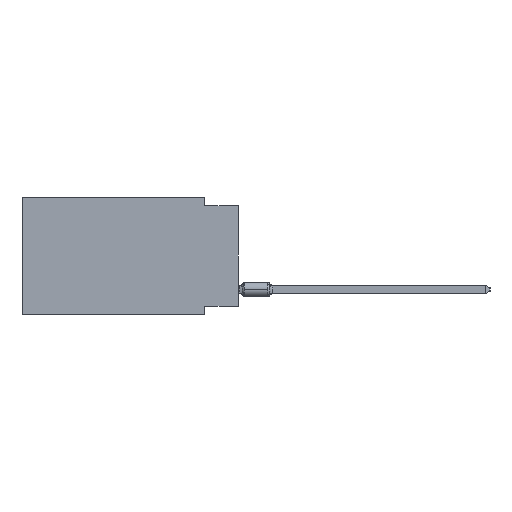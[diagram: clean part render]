
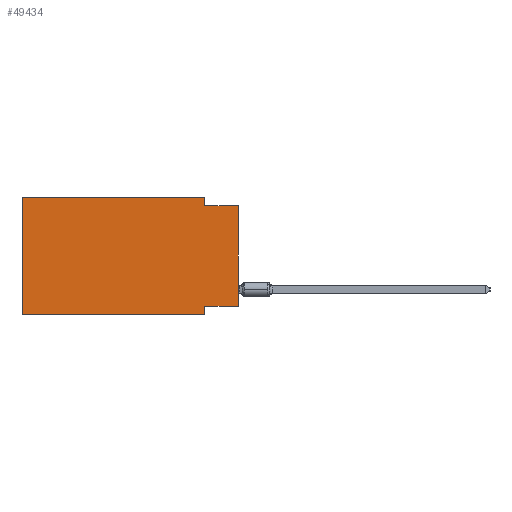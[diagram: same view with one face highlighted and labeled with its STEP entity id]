
A CAD part, left-side view. The second image highlights one B-rep face of the part: STEP entity #49434.
In plain terms, the highlighted planar face has unit normal (-1, 0, 0).
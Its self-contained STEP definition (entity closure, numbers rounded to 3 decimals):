
#2745 = DIRECTION ( 'NONE',  ( 0., -1., 0. ) ) ;
#3192 = ORIENTED_EDGE ( 'NONE', *, *, #61777, .T. ) ;
#5696 = ORIENTED_EDGE ( 'NONE', *, *, #51660, .F. ) ;
#6144 = VERTEX_POINT ( 'NONE', #36738 ) ;
#7599 = DIRECTION ( 'NONE',  ( 1., 0., 0. ) ) ;
#7860 = CARTESIAN_POINT ( 'NONE',  ( 0., 2.54, 0. ) ) ;
#9140 = CARTESIAN_POINT ( 'NONE',  ( 0., 2.54, -8.89 ) ) ;
#10076 = EDGE_CURVE ( 'NONE', #32012, #53193, #49525, .T. ) ;
#12968 = VECTOR ( 'NONE', #25764, 1000. ) ;
#13190 = AXIS2_PLACEMENT_3D ( 'NONE', #27248, #7599, #41908 ) ;
#13434 = LINE ( 'NONE', #22494, #43256 ) ;
#13563 = CARTESIAN_POINT ( 'NONE',  ( 0., 16.383, -8.89 ) ) ;
#13908 = CARTESIAN_POINT ( 'NONE',  ( 0., 0., -8.255 ) ) ;
#14457 = VECTOR ( 'NONE', #58638, 1000. ) ;
#14818 = DIRECTION ( 'NONE',  ( 0., -1., 0. ) ) ;
#14846 = LINE ( 'NONE', #33579, #31772 ) ;
#15227 = VERTEX_POINT ( 'NONE', #36261 ) ;
#16390 = VERTEX_POINT ( 'NONE', #13908 ) ;
#16767 = ORIENTED_EDGE ( 'NONE', *, *, #41672, .F. ) ;
#16909 = EDGE_CURVE ( 'NONE', #6144, #32012, #20112, .T. ) ;
#20112 = LINE ( 'NONE', #53565, #37125 ) ;
#20499 = CARTESIAN_POINT ( 'NONE',  ( 0., 0., -8.255 ) ) ;
#20774 = EDGE_CURVE ( 'NONE', #15227, #38412, #13434, .T. ) ;
#21414 = EDGE_CURVE ( 'NONE', #16390, #15227, #24565, .T. ) ;
#21467 = VECTOR ( 'NONE', #34677, 1000. ) ;
#22494 = CARTESIAN_POINT ( 'NONE',  ( 0., 2.54, -8.89 ) ) ;
#22847 = FACE_OUTER_BOUND ( 'NONE', #27957, .T. ) ;
#24565 = LINE ( 'NONE', #20499, #14457 ) ;
#25764 = DIRECTION ( 'NONE',  ( 0., 0., -1. ) ) ;
#27248 = CARTESIAN_POINT ( 'NONE',  ( 0., 16.383, 0. ) ) ;
#27957 = EDGE_LOOP ( 'NONE', ( #3192, #5696, #31625, #56081, #16767, #61664, #41090, #37866 ) ) ;
#31313 = DIRECTION ( 'NONE',  ( 0., 0., 1. ) ) ;
#31377 = CARTESIAN_POINT ( 'NONE',  ( 0., 16.383, -8.89 ) ) ;
#31625 = ORIENTED_EDGE ( 'NONE', *, *, #10076, .F. ) ;
#31772 = VECTOR ( 'NONE', #42969, 1000. ) ;
#31917 = PLANE ( 'NONE',  #13190 ) ;
#32012 = VERTEX_POINT ( 'NONE', #7860 ) ;
#33579 = CARTESIAN_POINT ( 'NONE',  ( 0., 0., -0.635 ) ) ;
#33860 = VECTOR ( 'NONE', #2745, 1000. ) ;
#34677 = DIRECTION ( 'NONE',  ( 0., 0., 1. ) ) ;
#35745 = CARTESIAN_POINT ( 'NONE',  ( 0., 2.54, 0. ) ) ;
#36261 = CARTESIAN_POINT ( 'NONE',  ( 0., 2.54, -8.255 ) ) ;
#36738 = CARTESIAN_POINT ( 'NONE',  ( 0., 16.383, 0. ) ) ;
#37125 = VECTOR ( 'NONE', #14818, 1000. ) ;
#37866 = ORIENTED_EDGE ( 'NONE', *, *, #21414, .F. ) ;
#38412 = VERTEX_POINT ( 'NONE', #9140 ) ;
#40692 = CARTESIAN_POINT ( 'NONE',  ( 0., 0., 0. ) ) ;
#40910 = VECTOR ( 'NONE', #31313, 1000. ) ;
#41090 = ORIENTED_EDGE ( 'NONE', *, *, #20774, .F. ) ;
#41672 = EDGE_CURVE ( 'NONE', #49804, #6144, #48441, .T. ) ;
#41908 = DIRECTION ( 'NONE',  ( 0., 0., -1. ) ) ;
#42969 = DIRECTION ( 'NONE',  ( 0., -1., 0. ) ) ;
#43256 = VECTOR ( 'NONE', #55942, 1000. ) ;
#44353 = CARTESIAN_POINT ( 'NONE',  ( 0., 16.383, 0. ) ) ;
#45091 = EDGE_CURVE ( 'NONE', #49804, #38412, #47283, .T. ) ;
#47137 = VERTEX_POINT ( 'NONE', #61657 ) ;
#47283 = LINE ( 'NONE', #13563, #33860 ) ;
#47431 = CARTESIAN_POINT ( 'NONE',  ( 0., 2.54, -0.635 ) ) ;
#48441 = LINE ( 'NONE', #44353, #21467 ) ;
#49434 = ADVANCED_FACE ( 'NONE', ( #22847 ), #31917, .F. ) ;
#49525 = LINE ( 'NONE', #35745, #12968 ) ;
#49804 = VERTEX_POINT ( 'NONE', #31377 ) ;
#51660 = EDGE_CURVE ( 'NONE', #53193, #47137, #14846, .T. ) ;
#53193 = VERTEX_POINT ( 'NONE', #47431 ) ;
#53565 = CARTESIAN_POINT ( 'NONE',  ( 0., 16.383, 0. ) ) ;
#55077 = LINE ( 'NONE', #40692, #40910 ) ;
#55942 = DIRECTION ( 'NONE',  ( 0., 0., -1. ) ) ;
#56081 = ORIENTED_EDGE ( 'NONE', *, *, #16909, .F. ) ;
#58638 = DIRECTION ( 'NONE',  ( 0., 1., 0. ) ) ;
#61657 = CARTESIAN_POINT ( 'NONE',  ( 0., 0., -0.635 ) ) ;
#61664 = ORIENTED_EDGE ( 'NONE', *, *, #45091, .T. ) ;
#61777 = EDGE_CURVE ( 'NONE', #16390, #47137, #55077, .T. ) ;
